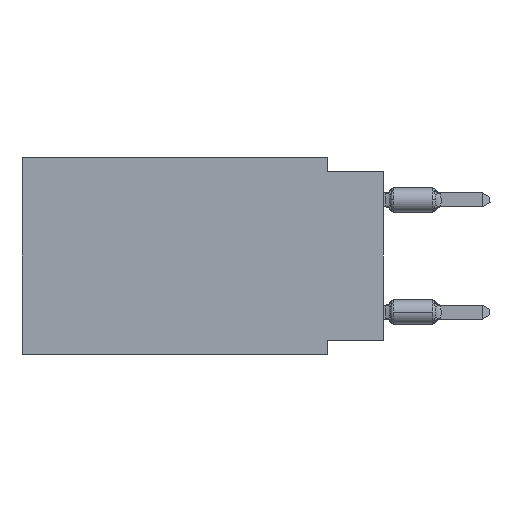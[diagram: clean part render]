
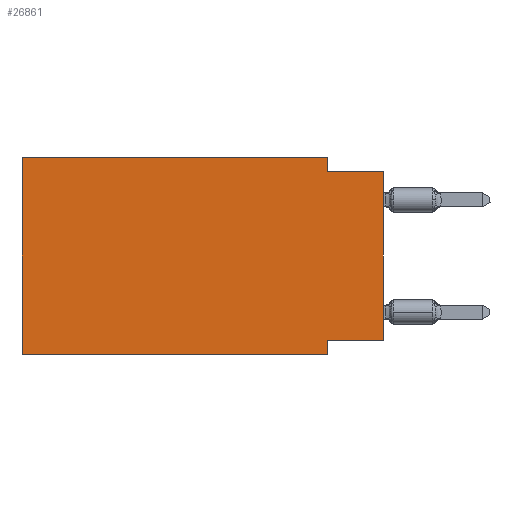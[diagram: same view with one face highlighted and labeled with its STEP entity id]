
A CAD part, left-side view. The second image highlights one B-rep face of the part: STEP entity #26861.
In plain terms, the highlighted planar face has unit normal (-1, 0, 0).
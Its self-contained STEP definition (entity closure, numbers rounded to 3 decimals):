
#312 = EDGE_CURVE ( 'NONE', #4867, #895, #26366, .T. ) ;
#725 = VECTOR ( 'NONE', #8792, 1000. ) ;
#895 = VERTEX_POINT ( 'NONE', #5217 ) ;
#1636 = CARTESIAN_POINT ( 'NONE',  ( 0., 16.383, 0. ) ) ;
#2763 = DIRECTION ( 'NONE',  ( 0., 0., 1. ) ) ;
#2871 = VECTOR ( 'NONE', #10817, 1000. ) ;
#2904 = ORIENTED_EDGE ( 'NONE', *, *, #29496, .T. ) ;
#3283 = EDGE_CURVE ( 'NONE', #16930, #23090, #30259, .T. ) ;
#3664 = ORIENTED_EDGE ( 'NONE', *, *, #23149, .T. ) ;
#4234 = ORIENTED_EDGE ( 'NONE', *, *, #29065, .F. ) ;
#4867 = VERTEX_POINT ( 'NONE', #5732 ) ;
#4890 = VECTOR ( 'NONE', #12859, 1000. ) ;
#5217 = CARTESIAN_POINT ( 'NONE',  ( 0., 2.54, -8.255 ) ) ;
#5245 = CARTESIAN_POINT ( 'NONE',  ( 0., 16.383, 0. ) ) ;
#5294 = LINE ( 'NONE', #19725, #22241 ) ;
#5732 = CARTESIAN_POINT ( 'NONE',  ( 0., 0., -8.255 ) ) ;
#5897 = VECTOR ( 'NONE', #25529, 1000. ) ;
#5966 = CARTESIAN_POINT ( 'NONE',  ( 0., 16.383, -8.89 ) ) ;
#7146 = DIRECTION ( 'NONE',  ( 0., 0., 1. ) ) ;
#7522 = CARTESIAN_POINT ( 'NONE',  ( 0., 2.54, 0. ) ) ;
#8568 = CARTESIAN_POINT ( 'NONE',  ( 0., 2.54, -8.89 ) ) ;
#8792 = DIRECTION ( 'NONE',  ( 0., 1., 0. ) ) ;
#8888 = VECTOR ( 'NONE', #13937, 1000. ) ;
#10817 = DIRECTION ( 'NONE',  ( 0., -1., 0. ) ) ;
#11040 = DIRECTION ( 'NONE',  ( 0., -1., 0. ) ) ;
#11353 = ORIENTED_EDGE ( 'NONE', *, *, #312, .F. ) ;
#12033 = EDGE_CURVE ( 'NONE', #12202, #17435, #12892, .T. ) ;
#12116 = ORIENTED_EDGE ( 'NONE', *, *, #12439, .F. ) ;
#12202 = VERTEX_POINT ( 'NONE', #25848 ) ;
#12439 = EDGE_CURVE ( 'NONE', #895, #26061, #24582, .T. ) ;
#12558 = LINE ( 'NONE', #5245, #29723 ) ;
#12561 = CARTESIAN_POINT ( 'NONE',  ( 0., 2.54, -8.89 ) ) ;
#12859 = DIRECTION ( 'NONE',  ( 0., 0., -1. ) ) ;
#12892 = LINE ( 'NONE', #15129, #2871 ) ;
#13276 = LINE ( 'NONE', #5966, #29632 ) ;
#13442 = EDGE_CURVE ( 'NONE', #21998, #16930, #12558, .T. ) ;
#13937 = DIRECTION ( 'NONE',  ( 0., 0., -1. ) ) ;
#15129 = CARTESIAN_POINT ( 'NONE',  ( 0., 0., -0.635 ) ) ;
#15880 = CARTESIAN_POINT ( 'NONE',  ( 0., 16.383, 0. ) ) ;
#16930 = VERTEX_POINT ( 'NONE', #1636 ) ;
#17435 = VERTEX_POINT ( 'NONE', #18615 ) ;
#18615 = CARTESIAN_POINT ( 'NONE',  ( 0., 0., -0.635 ) ) ;
#19725 = CARTESIAN_POINT ( 'NONE',  ( 0., 0., 0. ) ) ;
#19781 = EDGE_LOOP ( 'NONE', ( #3664, #28113, #4234, #23486, #22237, #2904, #12116, #11353 ) ) ;
#21887 = CARTESIAN_POINT ( 'NONE',  ( 0., 16.383, -8.89 ) ) ;
#21998 = VERTEX_POINT ( 'NONE', #21887 ) ;
#22237 = ORIENTED_EDGE ( 'NONE', *, *, #13442, .F. ) ;
#22241 = VECTOR ( 'NONE', #2763, 1000. ) ;
#23056 = CARTESIAN_POINT ( 'NONE',  ( 0., 16.383, 0. ) ) ;
#23090 = VERTEX_POINT ( 'NONE', #7522 ) ;
#23149 = EDGE_CURVE ( 'NONE', #4867, #17435, #5294, .T. ) ;
#23486 = ORIENTED_EDGE ( 'NONE', *, *, #3283, .F. ) ;
#24582 = LINE ( 'NONE', #12561, #4890 ) ;
#25115 = DIRECTION ( 'NONE',  ( 0., 0., -1. ) ) ;
#25529 = DIRECTION ( 'NONE',  ( 0., -1., 0. ) ) ;
#25583 = PLANE ( 'NONE',  #26805 ) ;
#25643 = LINE ( 'NONE', #30386, #8888 ) ;
#25848 = CARTESIAN_POINT ( 'NONE',  ( 0., 2.54, -0.635 ) ) ;
#26061 = VERTEX_POINT ( 'NONE', #8568 ) ;
#26366 = LINE ( 'NONE', #30470, #725 ) ;
#26805 = AXIS2_PLACEMENT_3D ( 'NONE', #23056, #30009, #25115 ) ;
#26861 = ADVANCED_FACE ( 'NONE', ( #27482 ), #25583, .F. ) ;
#27482 = FACE_OUTER_BOUND ( 'NONE', #19781, .T. ) ;
#28113 = ORIENTED_EDGE ( 'NONE', *, *, #12033, .F. ) ;
#29065 = EDGE_CURVE ( 'NONE', #23090, #12202, #25643, .T. ) ;
#29496 = EDGE_CURVE ( 'NONE', #21998, #26061, #13276, .T. ) ;
#29632 = VECTOR ( 'NONE', #11040, 1000. ) ;
#29723 = VECTOR ( 'NONE', #7146, 1000. ) ;
#30009 = DIRECTION ( 'NONE',  ( 1., 0., 0. ) ) ;
#30259 = LINE ( 'NONE', #15880, #5897 ) ;
#30386 = CARTESIAN_POINT ( 'NONE',  ( 0., 2.54, 0. ) ) ;
#30470 = CARTESIAN_POINT ( 'NONE',  ( 0., 0., -8.255 ) ) ;
